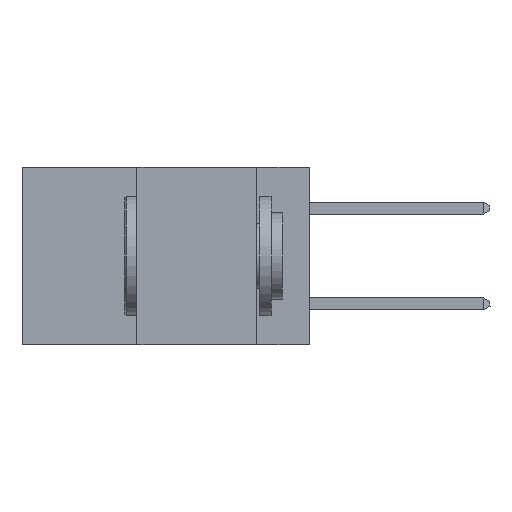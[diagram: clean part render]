
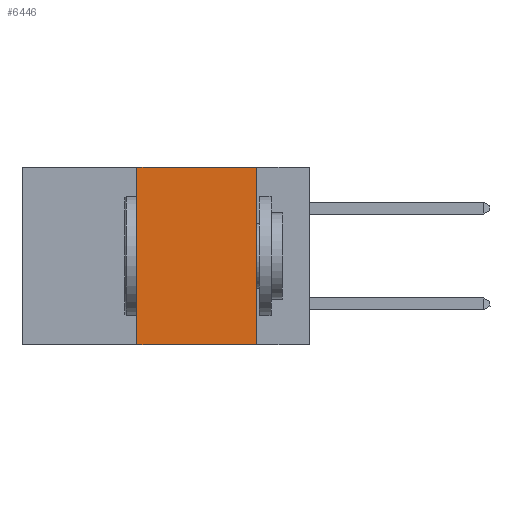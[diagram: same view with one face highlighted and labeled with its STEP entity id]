
A CAD part, left-side view. The second image highlights one B-rep face of the part: STEP entity #6446.
In plain terms, the highlighted planar face has unit normal (-1, 0, 0).
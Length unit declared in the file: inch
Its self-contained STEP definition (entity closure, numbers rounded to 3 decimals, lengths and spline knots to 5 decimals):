
#139 = ORIENTED_EDGE ( 'NONE', *, *, #8726, .F. ) ;
#191 = LINE ( 'NONE', #8045, #14222 ) ;
#339 = ORIENTED_EDGE ( 'NONE', *, *, #9325, .T. ) ;
#453 = VERTEX_POINT ( 'NONE', #15117 ) ;
#536 = LINE ( 'NONE', #13519, #4312 ) ;
#799 = CARTESIAN_POINT ( 'NONE',  ( 0., 0.6, 0. ) ) ;
#1212 = VECTOR ( 'NONE', #11355, 39.37008 ) ;
#1448 = ORIENTED_EDGE ( 'NONE', *, *, #14374, .F. ) ;
#1788 = CARTESIAN_POINT ( 'NONE',  ( 0., 0.36, 0. ) ) ;
#2111 = VECTOR ( 'NONE', #5496, 39.37008 ) ;
#2650 = DIRECTION ( 'NONE',  ( 0., 0., -1. ) ) ;
#3673 = DIRECTION ( 'NONE',  ( 1., 0., 0. ) ) ;
#4312 = VECTOR ( 'NONE', #14792, 39.37008 ) ;
#4953 = LINE ( 'NONE', #15222, #1212 ) ;
#5496 = DIRECTION ( 'NONE',  ( 0., 0., 1. ) ) ;
#6039 = CARTESIAN_POINT ( 'NONE',  ( 0., 0.36, -0.37 ) ) ;
#6446 = ADVANCED_FACE ( 'NONE', ( #14213 ), #7664, .F. ) ;
#7664 = PLANE ( 'NONE',  #11228 ) ;
#8045 = CARTESIAN_POINT ( 'NONE',  ( 0., 0.11, 0. ) ) ;
#8396 = EDGE_LOOP ( 'NONE', ( #15389, #1448, #139, #339 ) ) ;
#8726 = EDGE_CURVE ( 'NONE', #10230, #10877, #9790, .T. ) ;
#9325 = EDGE_CURVE ( 'NONE', #10230, #453, #536, .T. ) ;
#9790 = LINE ( 'NONE', #16172, #2111 ) ;
#10230 = VERTEX_POINT ( 'NONE', #6039 ) ;
#10331 = CARTESIAN_POINT ( 'NONE',  ( 0., 0.11, 0. ) ) ;
#10877 = VERTEX_POINT ( 'NONE', #1788 ) ;
#11228 = AXIS2_PLACEMENT_3D ( 'NONE', #799, #3673, #13033 ) ;
#11355 = DIRECTION ( 'NONE',  ( 0., -1., 0. ) ) ;
#13033 = DIRECTION ( 'NONE',  ( 0., 0., -1. ) ) ;
#13519 = CARTESIAN_POINT ( 'NONE',  ( 0., 0.6, -0.37 ) ) ;
#14213 = FACE_OUTER_BOUND ( 'NONE', #8396, .T. ) ;
#14222 = VECTOR ( 'NONE', #2650, 39.37008 ) ;
#14374 = EDGE_CURVE ( 'NONE', #10877, #16955, #4953, .T. ) ;
#14792 = DIRECTION ( 'NONE',  ( 0., -1., 0. ) ) ;
#15117 = CARTESIAN_POINT ( 'NONE',  ( 0., 0.11, -0.37 ) ) ;
#15222 = CARTESIAN_POINT ( 'NONE',  ( 0., 0.6, 0. ) ) ;
#15389 = ORIENTED_EDGE ( 'NONE', *, *, #15856, .F. ) ;
#15856 = EDGE_CURVE ( 'NONE', #16955, #453, #191, .T. ) ;
#16172 = CARTESIAN_POINT ( 'NONE',  ( 0., 0.36, 0. ) ) ;
#16955 = VERTEX_POINT ( 'NONE', #10331 ) ;
